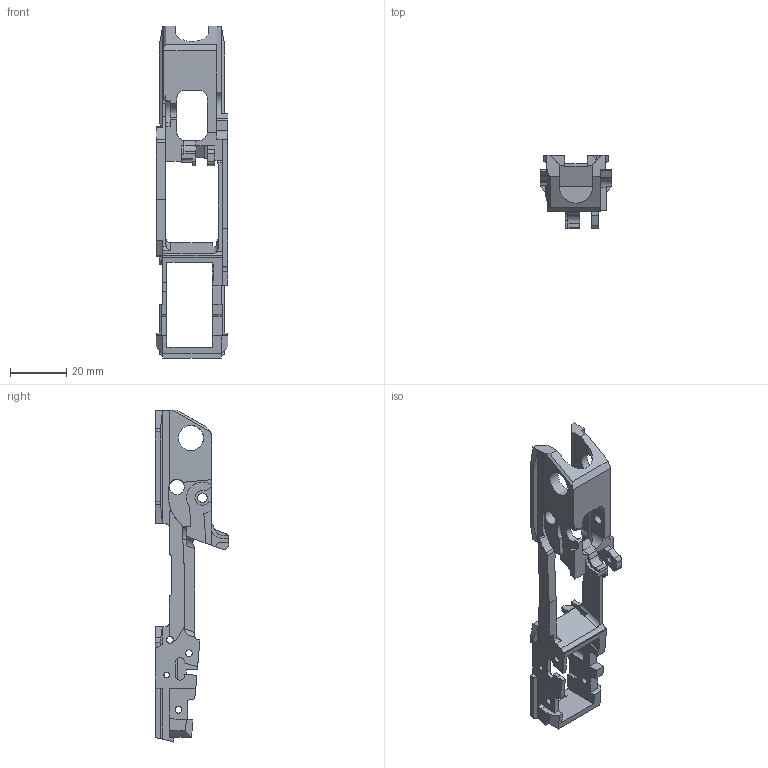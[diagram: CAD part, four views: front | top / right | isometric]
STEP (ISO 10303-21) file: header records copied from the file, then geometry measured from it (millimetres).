
FILE_DESCRIPTION(/* description */ (''),/* implementation_level */ '2;1');
FILE_NAME(/* name */ 'Ruger American Chassis.step',/* time_stamp */ '2019-10-25T18:27:29-04:00',/* author */ (''),/* organization */ (''),/* preprocessor_version */ 'ST-DEVELOPER v18',/* originating_system */ 'Autodesk Translation Framework v8.6.0.1094',/* authorisation */ '');
FILE_SCHEMA (('AUTOMOTIVE_DESIGN { 1 0 10303 214 3 1 1 }'));
Length unit declared in the file: millimetre
Products named in the file (1): Ruger American Chassis
Bounding box: 25.5 x 26 x 118 mm (x, y, z)
Volume: 11642.6 mm3; surface area: 10716.9 mm2
Topology: 1 solids, 1 shells, 257 faces, 767 edges, 506 vertices
Faces by surface type: plane 171, cylinder 83, sphere 2, torus 1
Full cylindrical faces by diameter (mm): 2 x1, 2.4 x9, 2.65 x1, 3.2 x2, 3.4 x1, 5.3 x2, 8.95 x1
Entity records: 8860 total; most frequent: CARTESIAN_POINT 1708, ORIENTED_EDGE 1534, DIRECTION 1448, EDGE_CURVE 767, LINE 570, VECTOR 570, VERTEX_POINT 506, AXIS2_PLACEMENT_3D 439
